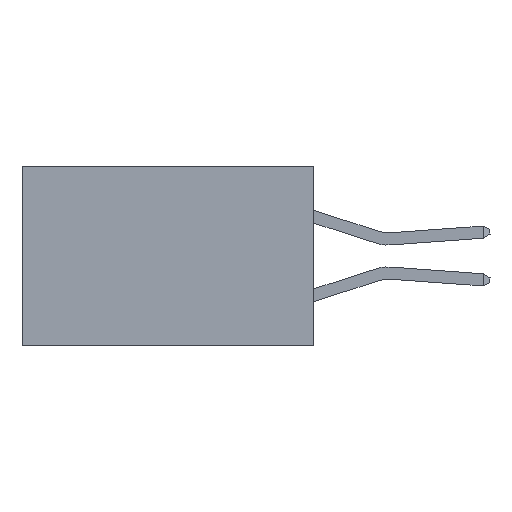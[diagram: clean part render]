
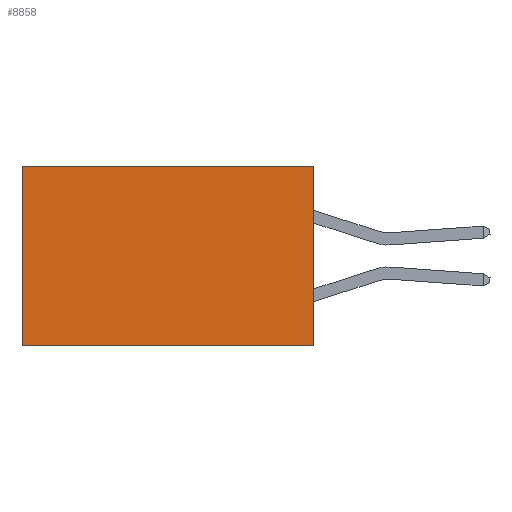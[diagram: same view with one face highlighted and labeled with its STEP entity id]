
A CAD part, left-side view. The second image highlights one B-rep face of the part: STEP entity #8858.
In plain terms, the highlighted planar face has unit normal (-1, 0, 0).
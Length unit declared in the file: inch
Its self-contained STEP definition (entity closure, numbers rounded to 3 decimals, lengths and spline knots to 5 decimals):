
#73 = CARTESIAN_POINT ( 'NONE',  ( 0.2875, 0.6, 0. ) ) ;
#254 = VERTEX_POINT ( 'NONE', #12561 ) ;
#2509 = VECTOR ( 'NONE', #9525, 39.37008 ) ;
#3813 = CARTESIAN_POINT ( 'NONE',  ( 0.2875, 0., 0. ) ) ;
#4367 = EDGE_CURVE ( 'NONE', #254, #30516, #9044, .T. ) ;
#5432 = ORIENTED_EDGE ( 'NONE', *, *, #15812, .F. ) ;
#6455 = DIRECTION ( 'NONE',  ( 0., 1., 0. ) ) ;
#7855 = LINE ( 'NONE', #3813, #26483 ) ;
#8858 = ADVANCED_FACE ( 'NONE', ( #27835 ), #19216, .F. ) ;
#8911 = DIRECTION ( 'NONE',  ( 0., 1., 0. ) ) ;
#9044 = LINE ( 'NONE', #73, #28100 ) ;
#9525 = DIRECTION ( 'NONE',  ( 0., 0., -1. ) ) ;
#9631 = ORIENTED_EDGE ( 'NONE', *, *, #19416, .F. ) ;
#12226 = VERTEX_POINT ( 'NONE', #26007 ) ;
#12561 = CARTESIAN_POINT ( 'NONE',  ( 0.2875, 0.6, 0. ) ) ;
#12632 = LINE ( 'NONE', #29181, #14568 ) ;
#13655 = CARTESIAN_POINT ( 'NONE',  ( 0.2875, 0.6, -0.37 ) ) ;
#13782 = DIRECTION ( 'NONE',  ( 1., 0., 0. ) ) ;
#14500 = CARTESIAN_POINT ( 'NONE',  ( 0.2875, 0., 0. ) ) ;
#14568 = VECTOR ( 'NONE', #6455, 39.37008 ) ;
#14630 = VERTEX_POINT ( 'NONE', #21996 ) ;
#15466 = DIRECTION ( 'NONE',  ( 0., 0., -1. ) ) ;
#15774 = AXIS2_PLACEMENT_3D ( 'NONE', #28970, #13782, #16543 ) ;
#15812 = EDGE_CURVE ( 'NONE', #12226, #14630, #17955, .T. ) ;
#16543 = DIRECTION ( 'NONE',  ( 0., 0., -1. ) ) ;
#17955 = LINE ( 'NONE', #14500, #2509 ) ;
#18836 = ORIENTED_EDGE ( 'NONE', *, *, #4367, .T. ) ;
#19216 = PLANE ( 'NONE',  #15774 ) ;
#19416 = EDGE_CURVE ( 'NONE', #14630, #30516, #12632, .T. ) ;
#21996 = CARTESIAN_POINT ( 'NONE',  ( 0.2875, 0., -0.37 ) ) ;
#25092 = EDGE_LOOP ( 'NONE', ( #18836, #9631, #5432, #32674 ) ) ;
#26007 = CARTESIAN_POINT ( 'NONE',  ( 0.2875, 0., 0. ) ) ;
#26483 = VECTOR ( 'NONE', #8911, 39.37008 ) ;
#27835 = FACE_OUTER_BOUND ( 'NONE', #25092, .T. ) ;
#28100 = VECTOR ( 'NONE', #15466, 39.37008 ) ;
#28970 = CARTESIAN_POINT ( 'NONE',  ( 0.2875, 0., 0. ) ) ;
#29181 = CARTESIAN_POINT ( 'NONE',  ( 0.2875, 0., -0.37 ) ) ;
#30516 = VERTEX_POINT ( 'NONE', #13655 ) ;
#32674 = ORIENTED_EDGE ( 'NONE', *, *, #32736, .T. ) ;
#32736 = EDGE_CURVE ( 'NONE', #12226, #254, #7855, .T. ) ;
